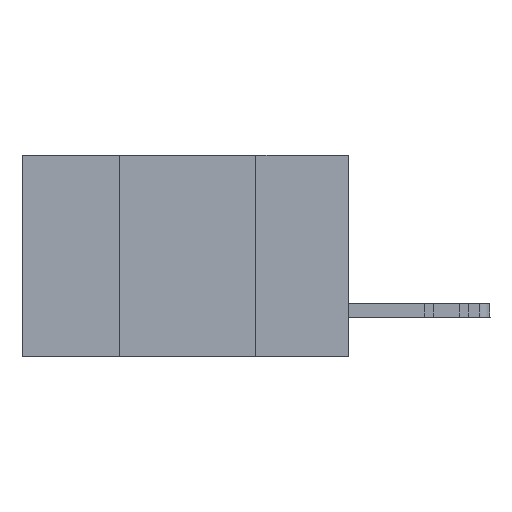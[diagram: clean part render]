
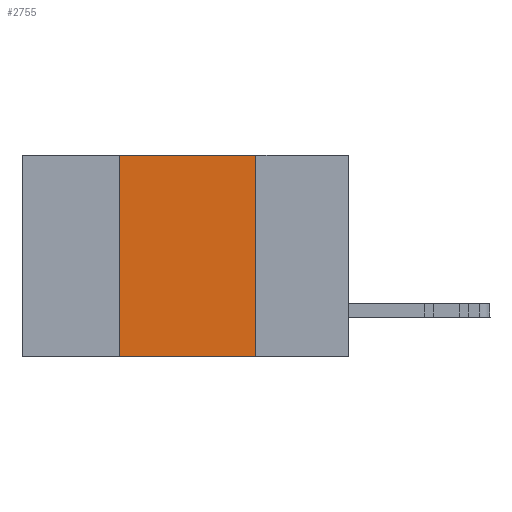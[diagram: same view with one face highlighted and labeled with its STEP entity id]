
A CAD part, left-side view. The second image highlights one B-rep face of the part: STEP entity #2755.
In plain terms, the highlighted planar face has unit normal (-1, 0, 0).
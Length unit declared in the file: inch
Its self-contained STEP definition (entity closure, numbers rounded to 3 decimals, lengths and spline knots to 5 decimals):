
#246 = VECTOR ( 'NONE', #7221, 39.37008 ) ;
#293 = LINE ( 'NONE', #9501, #23465 ) ;
#564 = EDGE_CURVE ( 'NONE', #19296, #26579, #12961, .T. ) ;
#668 = DIRECTION ( 'NONE',  ( 1., 0., 0. ) ) ;
#774 = DIRECTION ( 'NONE',  ( 0., -1., 0. ) ) ;
#1756 = ORIENTED_EDGE ( 'NONE', *, *, #564, .F. ) ;
#2755 = ADVANCED_FACE ( 'NONE', ( #13851 ), #4950, .F. ) ;
#2937 = DIRECTION ( 'NONE',  ( 0., 0., -1. ) ) ;
#3312 = DIRECTION ( 'NONE',  ( 0., 0., 1. ) ) ;
#3509 = CARTESIAN_POINT ( 'NONE',  ( 0., 0.42, 0. ) ) ;
#4950 = PLANE ( 'NONE',  #8010 ) ;
#5753 = CARTESIAN_POINT ( 'NONE',  ( 0., 0.42, 0. ) ) ;
#6863 = EDGE_CURVE ( 'NONE', #26265, #19296, #293, .T. ) ;
#7107 = CARTESIAN_POINT ( 'NONE',  ( 0., 0.6, 0. ) ) ;
#7221 = DIRECTION ( 'NONE',  ( 0., -1., 0. ) ) ;
#7733 = EDGE_CURVE ( 'NONE', #23924, #26579, #11452, .T. ) ;
#8010 = AXIS2_PLACEMENT_3D ( 'NONE', #7107, #668, #2937 ) ;
#8373 = CARTESIAN_POINT ( 'NONE',  ( 0., 0.17, -0.37 ) ) ;
#9501 = CARTESIAN_POINT ( 'NONE',  ( 0., 0.6, 0. ) ) ;
#11452 = LINE ( 'NONE', #15736, #246 ) ;
#12183 = VECTOR ( 'NONE', #3312, 39.37008 ) ;
#12471 = EDGE_CURVE ( 'NONE', #23924, #26265, #22424, .T. ) ;
#12645 = ORIENTED_EDGE ( 'NONE', *, *, #7733, .T. ) ;
#12834 = EDGE_LOOP ( 'NONE', ( #1756, #23359, #25001, #12645 ) ) ;
#12961 = LINE ( 'NONE', #15726, #18088 ) ;
#13851 = FACE_OUTER_BOUND ( 'NONE', #12834, .T. ) ;
#15726 = CARTESIAN_POINT ( 'NONE',  ( 0., 0.17, 0. ) ) ;
#15736 = CARTESIAN_POINT ( 'NONE',  ( 0., 0.6, -0.37 ) ) ;
#16609 = CARTESIAN_POINT ( 'NONE',  ( 0., 0.42, -0.37 ) ) ;
#18088 = VECTOR ( 'NONE', #25244, 39.37008 ) ;
#19296 = VERTEX_POINT ( 'NONE', #25068 ) ;
#22424 = LINE ( 'NONE', #3509, #12183 ) ;
#23359 = ORIENTED_EDGE ( 'NONE', *, *, #6863, .F. ) ;
#23465 = VECTOR ( 'NONE', #774, 39.37008 ) ;
#23924 = VERTEX_POINT ( 'NONE', #16609 ) ;
#25001 = ORIENTED_EDGE ( 'NONE', *, *, #12471, .F. ) ;
#25068 = CARTESIAN_POINT ( 'NONE',  ( 0., 0.17, 0. ) ) ;
#25244 = DIRECTION ( 'NONE',  ( 0., 0., -1. ) ) ;
#26265 = VERTEX_POINT ( 'NONE', #5753 ) ;
#26579 = VERTEX_POINT ( 'NONE', #8373 ) ;
